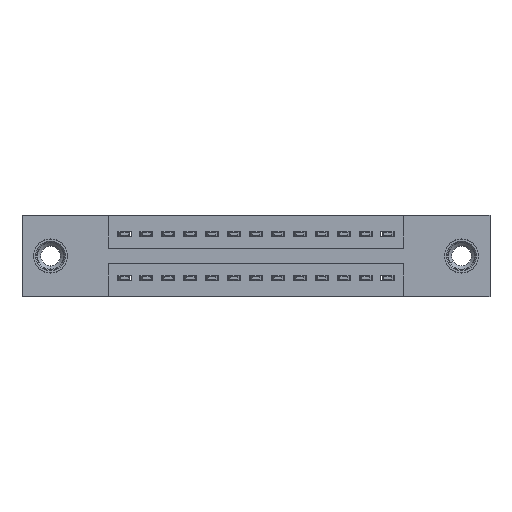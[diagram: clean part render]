
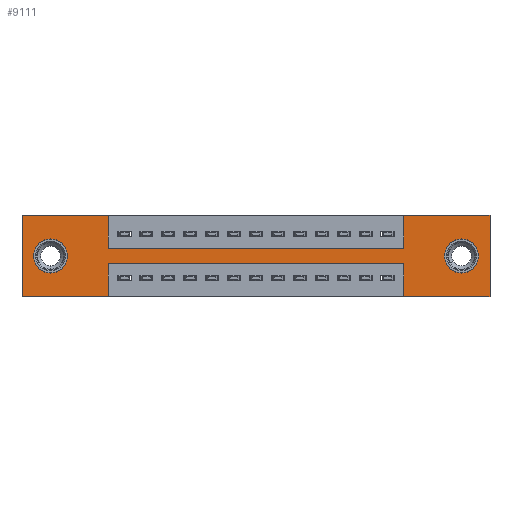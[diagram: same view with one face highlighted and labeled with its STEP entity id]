
A CAD part, front view. The second image highlights one B-rep face of the part: STEP entity #9111.
In plain terms, the highlighted planar face has unit normal (0, -1, 0).
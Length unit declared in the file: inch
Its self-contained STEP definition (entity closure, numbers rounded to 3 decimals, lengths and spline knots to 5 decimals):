
#265 = VECTOR ( 'NONE', #6300, 39.37008 ) ;
#282 = CARTESIAN_POINT ( 'NONE',  ( 0.13, 0., -0.263 ) ) ;
#382 = LINE ( 'NONE', #1581, #12448 ) ;
#439 = CIRCLE ( 'NONE', #13735, 0.078 ) ;
#516 = CARTESIAN_POINT ( 'NONE',  ( 0.13, 0., -0.185 ) ) ;
#653 = VECTOR ( 'NONE', #8758, 39.37008 ) ;
#724 = VERTEX_POINT ( 'NONE', #1134 ) ;
#746 = VERTEX_POINT ( 'NONE', #2072 ) ;
#798 = DIRECTION ( 'NONE',  ( 1., 0., 0. ) ) ;
#841 = DIRECTION ( 'NONE',  ( 0., 0., -1. ) ) ;
#1134 = CARTESIAN_POINT ( 'NONE',  ( 0.3925, 0., -0.37 ) ) ;
#1201 = VECTOR ( 'NONE', #4346, 39.37008 ) ;
#1208 = CARTESIAN_POINT ( 'NONE',  ( 2.135, 0., -0.37 ) ) ;
#1581 = CARTESIAN_POINT ( 'NONE',  ( 0., 0., 0. ) ) ;
#1631 = CARTESIAN_POINT ( 'NONE',  ( 2.005, 0., -0.107 ) ) ;
#1774 = DIRECTION ( 'NONE',  ( 0., 0., 1. ) ) ;
#1829 = CARTESIAN_POINT ( 'NONE',  ( 0.3925, 0., 0. ) ) ;
#2070 = CARTESIAN_POINT ( 'NONE',  ( 2.135, 0., 0. ) ) ;
#2072 = CARTESIAN_POINT ( 'NONE',  ( 0.3925, 0., -0.15 ) ) ;
#2147 = DIRECTION ( 'NONE',  ( 0., 0., 1. ) ) ;
#2171 = VECTOR ( 'NONE', #2716, 39.37008 ) ;
#2378 = VECTOR ( 'NONE', #798, 39.37008 ) ;
#2639 = VERTEX_POINT ( 'NONE', #8434 ) ;
#2716 = DIRECTION ( 'NONE',  ( 0., 0., -1. ) ) ;
#2998 = VERTEX_POINT ( 'NONE', #1208 ) ;
#3016 = EDGE_CURVE ( 'NONE', #724, #10249, #13994, .T. ) ;
#3117 = VECTOR ( 'NONE', #11640, 39.37008 ) ;
#3150 = EDGE_LOOP ( 'NONE', ( #4220, #4247, #4347, #4378, #4403, #4434, #4464, #4525, #4541, #4585, #4803, #5028 ) ) ;
#3194 = EDGE_LOOP ( 'NONE', ( #4118, #4156 ) ) ;
#3342 = CARTESIAN_POINT ( 'NONE',  ( 0., 0., -0.37 ) ) ;
#3419 = CARTESIAN_POINT ( 'NONE',  ( 1.7425, 0., -0.37 ) ) ;
#3424 = CARTESIAN_POINT ( 'NONE',  ( 0.3925, 0., -0.22 ) ) ;
#3725 = LINE ( 'NONE', #2070, #6411 ) ;
#3845 = LINE ( 'NONE', #6438, #653 ) ;
#3873 = VERTEX_POINT ( 'NONE', #282 ) ;
#3992 = ORIENTED_EDGE ( 'NONE', *, *, #14859, .T. ) ;
#4016 = DIRECTION ( 'NONE',  ( 0., 1., 0. ) ) ;
#4107 = ORIENTED_EDGE ( 'NONE', *, *, #7391, .T. ) ;
#4118 = ORIENTED_EDGE ( 'NONE', *, *, #13573, .T. ) ;
#4156 = ORIENTED_EDGE ( 'NONE', *, *, #6707, .T. ) ;
#4203 = CARTESIAN_POINT ( 'NONE',  ( 2.135, 0., 0. ) ) ;
#4220 = ORIENTED_EDGE ( 'NONE', *, *, #14103, .F. ) ;
#4247 = ORIENTED_EDGE ( 'NONE', *, *, #13315, .F. ) ;
#4346 = DIRECTION ( 'NONE',  ( -1., 0., 0. ) ) ;
#4347 = ORIENTED_EDGE ( 'NONE', *, *, #12575, .F. ) ;
#4378 = ORIENTED_EDGE ( 'NONE', *, *, #6084, .F. ) ;
#4403 = ORIENTED_EDGE ( 'NONE', *, *, #8406, .F. ) ;
#4434 = ORIENTED_EDGE ( 'NONE', *, *, #11182, .F. ) ;
#4464 = ORIENTED_EDGE ( 'NONE', *, *, #11808, .F. ) ;
#4470 = CARTESIAN_POINT ( 'NONE',  ( 1.7425, 0., -0.15 ) ) ;
#4525 = ORIENTED_EDGE ( 'NONE', *, *, #11042, .F. ) ;
#4541 = ORIENTED_EDGE ( 'NONE', *, *, #9475, .F. ) ;
#4585 = ORIENTED_EDGE ( 'NONE', *, *, #14840, .F. ) ;
#4719 = VECTOR ( 'NONE', #2147, 39.37008 ) ;
#4803 = ORIENTED_EDGE ( 'NONE', *, *, #12284, .F. ) ;
#5028 = ORIENTED_EDGE ( 'NONE', *, *, #3016, .F. ) ;
#5078 = DIRECTION ( 'NONE',  ( 0., 1., 0. ) ) ;
#5090 = CIRCLE ( 'NONE', #11572, 0.078 ) ;
#5100 = CARTESIAN_POINT ( 'NONE',  ( 0.13, 0., -0.107 ) ) ;
#5141 = DIRECTION ( 'NONE',  ( 1., 0., 0. ) ) ;
#5423 = CARTESIAN_POINT ( 'NONE',  ( 0., 0., 0. ) ) ;
#5515 = FACE_BOUND ( 'NONE', #3194, .T. ) ;
#5733 = CARTESIAN_POINT ( 'NONE',  ( 1.7425, 0., 0. ) ) ;
#5848 = FACE_OUTER_BOUND ( 'NONE', #3150, .T. ) ;
#5902 = CARTESIAN_POINT ( 'NONE',  ( 0., 0., -0.37 ) ) ;
#6084 = EDGE_CURVE ( 'NONE', #2998, #9790, #10133, .T. ) ;
#6224 = VERTEX_POINT ( 'NONE', #5733 ) ;
#6259 = CARTESIAN_POINT ( 'NONE',  ( 0., 0., 0. ) ) ;
#6300 = DIRECTION ( 'NONE',  ( 0., 0., -1. ) ) ;
#6411 = VECTOR ( 'NONE', #841, 39.37008 ) ;
#6416 = AXIS2_PLACEMENT_3D ( 'NONE', #10930, #4016, #12076 ) ;
#6438 = CARTESIAN_POINT ( 'NONE',  ( 0.3925, 0., -0.15 ) ) ;
#6561 = DIRECTION ( 'NONE',  ( 0., 1., 0. ) ) ;
#6707 = EDGE_CURVE ( 'NONE', #3873, #11580, #5090, .T. ) ;
#6789 = PLANE ( 'NONE',  #9259 ) ;
#6797 = AXIS2_PLACEMENT_3D ( 'NONE', #11965, #5078, #13093 ) ;
#7165 = VERTEX_POINT ( 'NONE', #1631 ) ;
#7354 = EDGE_LOOP ( 'NONE', ( #3992, #4107 ) ) ;
#7390 = DIRECTION ( 'NONE',  ( 0., 0., 1. ) ) ;
#7391 = EDGE_CURVE ( 'NONE', #2639, #7165, #14030, .T. ) ;
#7857 = VERTEX_POINT ( 'NONE', #3424 ) ;
#7894 = CARTESIAN_POINT ( 'NONE',  ( 1.7425, 0., -0.37 ) ) ;
#7938 = LINE ( 'NONE', #10796, #2171 ) ;
#7955 = DIRECTION ( 'NONE',  ( 0., 0., -1. ) ) ;
#8114 = VERTEX_POINT ( 'NONE', #11945 ) ;
#8289 = VECTOR ( 'NONE', #7390, 39.37008 ) ;
#8406 = EDGE_CURVE ( 'NONE', #11079, #2998, #3725, .T. ) ;
#8434 = CARTESIAN_POINT ( 'NONE',  ( 2.005, 0., -0.263 ) ) ;
#8587 = VECTOR ( 'NONE', #15114, 39.37008 ) ;
#8718 = DIRECTION ( 'NONE',  ( 0., 1., 0. ) ) ;
#8758 = DIRECTION ( 'NONE',  ( 1., 0., 0. ) ) ;
#8909 = CARTESIAN_POINT ( 'NONE',  ( 0., 0., 0. ) ) ;
#9048 = LINE ( 'NONE', #12281, #14786 ) ;
#9111 = ADVANCED_FACE ( 'NONE', ( #11284, #5515, #5848 ), #6789, .T. ) ;
#9259 = AXIS2_PLACEMENT_3D ( 'NONE', #3342, #14857, #7955 ) ;
#9387 = CIRCLE ( 'NONE', #6416, 0.078 ) ;
#9475 = EDGE_CURVE ( 'NONE', #13617, #746, #12690, .T. ) ;
#9790 = VERTEX_POINT ( 'NONE', #3419 ) ;
#10133 = LINE ( 'NONE', #12393, #1201 ) ;
#10249 = VERTEX_POINT ( 'NONE', #14488 ) ;
#10483 = CARTESIAN_POINT ( 'NONE',  ( 0.3925, 0., -0.22 ) ) ;
#10581 = VERTEX_POINT ( 'NONE', #5423 ) ;
#10796 = CARTESIAN_POINT ( 'NONE',  ( 0.3925, 0., -0.37 ) ) ;
#10930 = CARTESIAN_POINT ( 'NONE',  ( 2.005, 0., -0.185 ) ) ;
#11042 = EDGE_CURVE ( 'NONE', #746, #12559, #3845, .T. ) ;
#11079 = VERTEX_POINT ( 'NONE', #4203 ) ;
#11182 = EDGE_CURVE ( 'NONE', #6224, #11079, #11609, .T. ) ;
#11284 = FACE_BOUND ( 'NONE', #7354, .T. ) ;
#11572 = AXIS2_PLACEMENT_3D ( 'NONE', #13466, #6561, #14617 ) ;
#11580 = VERTEX_POINT ( 'NONE', #5100 ) ;
#11609 = LINE ( 'NONE', #8909, #2378 ) ;
#11640 = DIRECTION ( 'NONE',  ( -1., 0., 0. ) ) ;
#11748 = LINE ( 'NONE', #6259, #8289 ) ;
#11808 = EDGE_CURVE ( 'NONE', #12559, #6224, #9048, .T. ) ;
#11945 = CARTESIAN_POINT ( 'NONE',  ( 1.7425, 0., -0.22 ) ) ;
#11964 = LINE ( 'NONE', #10483, #3117 ) ;
#11965 = CARTESIAN_POINT ( 'NONE',  ( 2.005, 0., -0.185 ) ) ;
#12058 = CARTESIAN_POINT ( 'NONE',  ( 0.3925, 0., 0. ) ) ;
#12076 = DIRECTION ( 'NONE',  ( 0., 0., -1. ) ) ;
#12281 = CARTESIAN_POINT ( 'NONE',  ( 1.7425, 0., 0. ) ) ;
#12284 = EDGE_CURVE ( 'NONE', #10249, #10581, #11748, .T. ) ;
#12332 = DIRECTION ( 'NONE',  ( 0., 0., 1. ) ) ;
#12393 = CARTESIAN_POINT ( 'NONE',  ( 0., 0., -0.37 ) ) ;
#12448 = VECTOR ( 'NONE', #5141, 39.37008 ) ;
#12559 = VERTEX_POINT ( 'NONE', #4470 ) ;
#12575 = EDGE_CURVE ( 'NONE', #9790, #8114, #13881, .T. ) ;
#12690 = LINE ( 'NONE', #12058, #265 ) ;
#13093 = DIRECTION ( 'NONE',  ( 0., 0., -1. ) ) ;
#13315 = EDGE_CURVE ( 'NONE', #8114, #7857, #11964, .T. ) ;
#13466 = CARTESIAN_POINT ( 'NONE',  ( 0.13, 0., -0.185 ) ) ;
#13573 = EDGE_CURVE ( 'NONE', #11580, #3873, #439, .T. ) ;
#13617 = VERTEX_POINT ( 'NONE', #1829 ) ;
#13735 = AXIS2_PLACEMENT_3D ( 'NONE', #516, #8718, #1774 ) ;
#13881 = LINE ( 'NONE', #7894, #4719 ) ;
#13994 = LINE ( 'NONE', #5902, #8587 ) ;
#14030 = CIRCLE ( 'NONE', #6797, 0.078 ) ;
#14103 = EDGE_CURVE ( 'NONE', #7857, #724, #7938, .T. ) ;
#14488 = CARTESIAN_POINT ( 'NONE',  ( 0., 0., -0.37 ) ) ;
#14617 = DIRECTION ( 'NONE',  ( 0., 0., 1. ) ) ;
#14786 = VECTOR ( 'NONE', #12332, 39.37008 ) ;
#14840 = EDGE_CURVE ( 'NONE', #10581, #13617, #382, .T. ) ;
#14857 = DIRECTION ( 'NONE',  ( 0., -1., 0. ) ) ;
#14859 = EDGE_CURVE ( 'NONE', #7165, #2639, #9387, .T. ) ;
#15114 = DIRECTION ( 'NONE',  ( -1., 0., 0. ) ) ;
